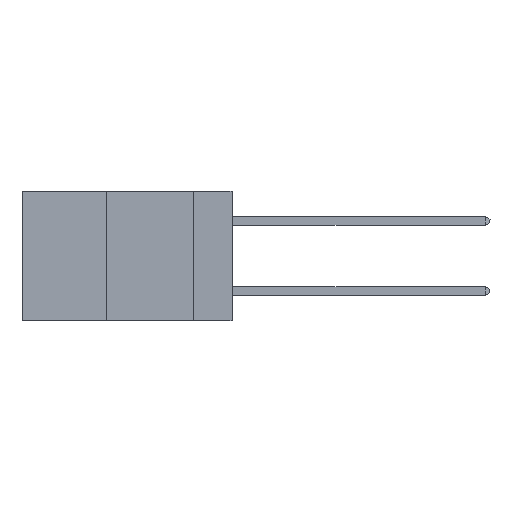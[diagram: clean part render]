
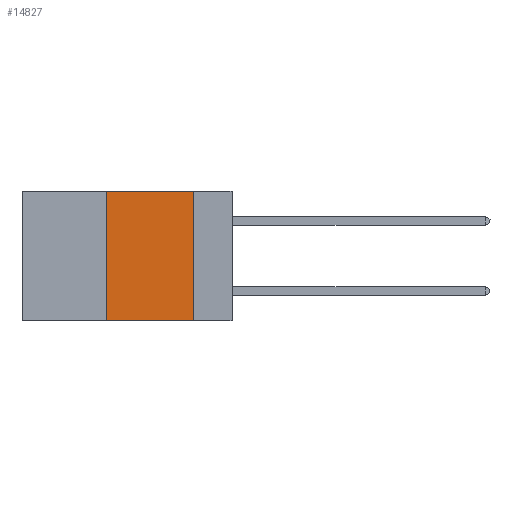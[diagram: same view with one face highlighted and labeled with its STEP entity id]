
A CAD part, left-side view. The second image highlights one B-rep face of the part: STEP entity #14827.
In plain terms, the highlighted planar face has unit normal (-1, 0, 0).
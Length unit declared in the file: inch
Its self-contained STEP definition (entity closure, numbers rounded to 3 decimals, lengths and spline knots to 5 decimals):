
#885 = EDGE_CURVE ( 'NONE', #37151, #43928, #43613, .T. ) ;
#1297 = DIRECTION ( 'NONE',  ( 0., -1., 0. ) ) ;
#2024 = VECTOR ( 'NONE', #1297, 39.37008 ) ;
#2531 = CARTESIAN_POINT ( 'NONE',  ( 0., 0.11, 0. ) ) ;
#3967 = CARTESIAN_POINT ( 'NONE',  ( 0., 0.11, -0.37 ) ) ;
#4301 = CARTESIAN_POINT ( 'NONE',  ( 0., 0.6, 0. ) ) ;
#7546 = ORIENTED_EDGE ( 'NONE', *, *, #45199, .F. ) ;
#7640 = CARTESIAN_POINT ( 'NONE',  ( 0., 0.36, -0.37 ) ) ;
#8041 = ORIENTED_EDGE ( 'NONE', *, *, #11395, .F. ) ;
#8769 = FACE_OUTER_BOUND ( 'NONE', #45395, .T. ) ;
#9447 = LINE ( 'NONE', #17383, #18013 ) ;
#9947 = ORIENTED_EDGE ( 'NONE', *, *, #885, .F. ) ;
#11395 = EDGE_CURVE ( 'NONE', #15059, #14723, #17073, .T. ) ;
#14170 = VECTOR ( 'NONE', #46232, 39.37008 ) ;
#14723 = VERTEX_POINT ( 'NONE', #3967 ) ;
#14827 = ADVANCED_FACE ( 'NONE', ( #8769 ), #15597, .F. ) ;
#15059 = VERTEX_POINT ( 'NONE', #27876 ) ;
#15597 = PLANE ( 'NONE',  #16157 ) ;
#15936 = CARTESIAN_POINT ( 'NONE',  ( 0., 0.36, 0. ) ) ;
#16157 = AXIS2_PLACEMENT_3D ( 'NONE', #34045, #19463, #33899 ) ;
#17073 = LINE ( 'NONE', #2531, #14170 ) ;
#17383 = CARTESIAN_POINT ( 'NONE',  ( 0., 0.6, -0.37 ) ) ;
#18013 = VECTOR ( 'NONE', #31553, 39.37008 ) ;
#19463 = DIRECTION ( 'NONE',  ( 1., 0., 0. ) ) ;
#24273 = EDGE_CURVE ( 'NONE', #37151, #14723, #9447, .T. ) ;
#27876 = CARTESIAN_POINT ( 'NONE',  ( 0., 0.11, 0. ) ) ;
#31553 = DIRECTION ( 'NONE',  ( 0., -1., 0. ) ) ;
#33899 = DIRECTION ( 'NONE',  ( 0., 0., -1. ) ) ;
#34045 = CARTESIAN_POINT ( 'NONE',  ( 0., 0.6, 0. ) ) ;
#37151 = VERTEX_POINT ( 'NONE', #7640 ) ;
#40179 = VECTOR ( 'NONE', #43558, 39.37008 ) ;
#41440 = ORIENTED_EDGE ( 'NONE', *, *, #24273, .T. ) ;
#43401 = CARTESIAN_POINT ( 'NONE',  ( 0., 0.36, 0. ) ) ;
#43532 = LINE ( 'NONE', #4301, #2024 ) ;
#43558 = DIRECTION ( 'NONE',  ( 0., 0., 1. ) ) ;
#43613 = LINE ( 'NONE', #43401, #40179 ) ;
#43928 = VERTEX_POINT ( 'NONE', #15936 ) ;
#45199 = EDGE_CURVE ( 'NONE', #43928, #15059, #43532, .T. ) ;
#45395 = EDGE_LOOP ( 'NONE', ( #8041, #7546, #9947, #41440 ) ) ;
#46232 = DIRECTION ( 'NONE',  ( 0., 0., -1. ) ) ;
